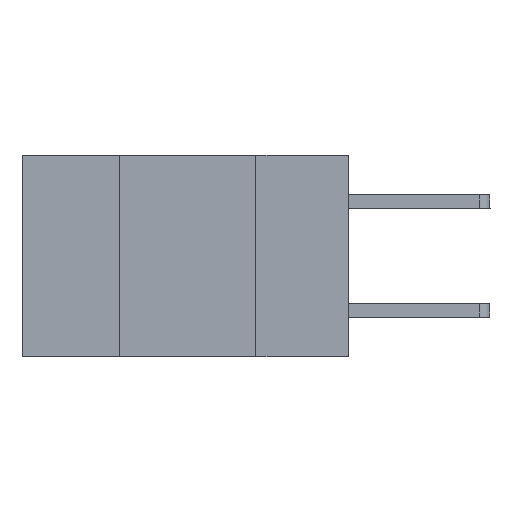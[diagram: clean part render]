
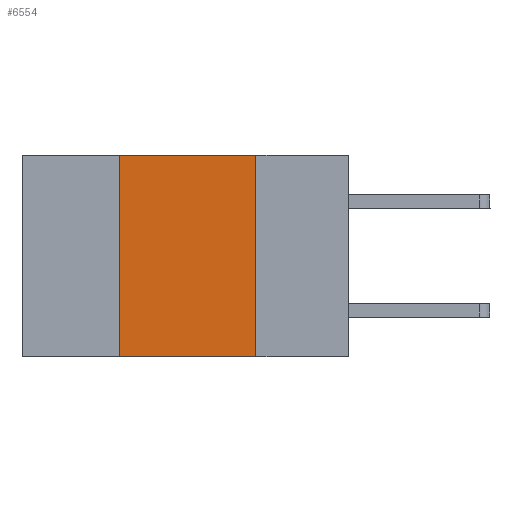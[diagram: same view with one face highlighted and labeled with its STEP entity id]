
A CAD part, left-side view. The second image highlights one B-rep face of the part: STEP entity #6554.
In plain terms, the highlighted planar face has unit normal (-1, 0, 0).
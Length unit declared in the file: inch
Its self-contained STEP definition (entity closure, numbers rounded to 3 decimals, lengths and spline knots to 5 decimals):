
#193 = DIRECTION ( 'NONE',  ( 1., 0., 0. ) ) ;
#622 = ORIENTED_EDGE ( 'NONE', *, *, #8075, .F. ) ;
#822 = CARTESIAN_POINT ( 'NONE',  ( 0., 0.17, 0. ) ) ;
#1629 = VERTEX_POINT ( 'NONE', #3154 ) ;
#2246 = AXIS2_PLACEMENT_3D ( 'NONE', #4991, #193, #4940 ) ;
#2579 = FACE_OUTER_BOUND ( 'NONE', #10029, .T. ) ;
#2716 = LINE ( 'NONE', #5168, #4053 ) ;
#2841 = ORIENTED_EDGE ( 'NONE', *, *, #9809, .T. ) ;
#3111 = CARTESIAN_POINT ( 'NONE',  ( 0., 0.6, -0.37 ) ) ;
#3140 = ORIENTED_EDGE ( 'NONE', *, *, #6448, .F. ) ;
#3154 = CARTESIAN_POINT ( 'NONE',  ( 0., 0.42, -0.37 ) ) ;
#4053 = VECTOR ( 'NONE', #8899, 39.37008 ) ;
#4095 = CARTESIAN_POINT ( 'NONE',  ( 0., 0.17, 0. ) ) ;
#4593 = LINE ( 'NONE', #822, #4879 ) ;
#4836 = PLANE ( 'NONE',  #2246 ) ;
#4879 = VECTOR ( 'NONE', #5406, 39.37008 ) ;
#4940 = DIRECTION ( 'NONE',  ( 0., 0., -1. ) ) ;
#4991 = CARTESIAN_POINT ( 'NONE',  ( 0., 0.6, 0. ) ) ;
#5168 = CARTESIAN_POINT ( 'NONE',  ( 0., 0.6, 0. ) ) ;
#5406 = DIRECTION ( 'NONE',  ( 0., 0., -1. ) ) ;
#6429 = VERTEX_POINT ( 'NONE', #7822 ) ;
#6448 = EDGE_CURVE ( 'NONE', #1629, #6774, #9332, .T. ) ;
#6554 = ADVANCED_FACE ( 'NONE', ( #2579 ), #4836, .F. ) ;
#6774 = VERTEX_POINT ( 'NONE', #9689 ) ;
#6931 = VECTOR ( 'NONE', #7058, 39.37008 ) ;
#7058 = DIRECTION ( 'NONE',  ( 0., 0., 1. ) ) ;
#7168 = VECTOR ( 'NONE', #7578, 39.37008 ) ;
#7578 = DIRECTION ( 'NONE',  ( 0., -1., 0. ) ) ;
#7622 = CARTESIAN_POINT ( 'NONE',  ( 0., 0.42, 0. ) ) ;
#7822 = CARTESIAN_POINT ( 'NONE',  ( 0., 0.17, -0.37 ) ) ;
#7950 = VERTEX_POINT ( 'NONE', #4095 ) ;
#8075 = EDGE_CURVE ( 'NONE', #6774, #7950, #2716, .T. ) ;
#8150 = EDGE_CURVE ( 'NONE', #7950, #6429, #4593, .T. ) ;
#8899 = DIRECTION ( 'NONE',  ( 0., -1., 0. ) ) ;
#9290 = LINE ( 'NONE', #3111, #7168 ) ;
#9332 = LINE ( 'NONE', #7622, #6931 ) ;
#9618 = ORIENTED_EDGE ( 'NONE', *, *, #8150, .F. ) ;
#9689 = CARTESIAN_POINT ( 'NONE',  ( 0., 0.42, 0. ) ) ;
#9809 = EDGE_CURVE ( 'NONE', #1629, #6429, #9290, .T. ) ;
#10029 = EDGE_LOOP ( 'NONE', ( #9618, #622, #3140, #2841 ) ) ;
